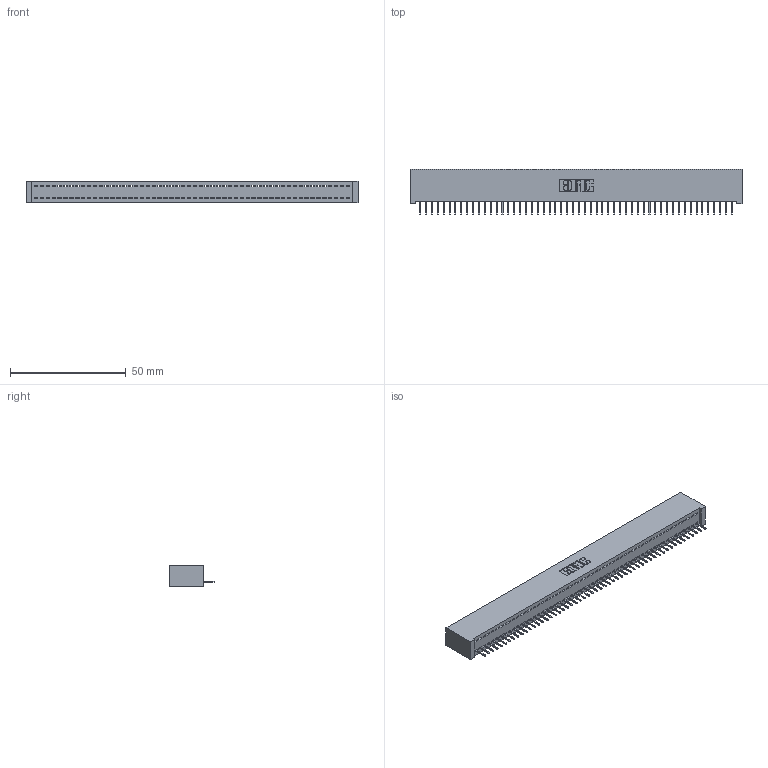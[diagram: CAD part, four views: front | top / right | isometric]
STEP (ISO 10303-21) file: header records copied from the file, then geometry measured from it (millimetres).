
FILE_DESCRIPTION (( 'STEP AP203' ), '1' );
FILE_NAME ('342-054-524-101.STEP', '2019-10-03T02:57:07', ( '' ), ( '' ), 'SwSTEP 2.0', 'SolidWorks 2016', '' );
FILE_SCHEMA (( 'CONFIG_CONTROL_DESIGN' ));
Length unit declared in the file: inch
Products named in the file (3): 342 Part_Lugless; 345-292-001_345-293-124; 342-054-524-101
Assembly tree (55 placements, depth 2):
  342-054-524-101
    342 Part_Lugless
    345-292-001_345-293-124  x54
Bounding box: 143.41 x 19.69 x 9.4 mm (x, y, z)
Volume: 12813.9 mm3; surface area: 18701.4 mm2
Topology: 55 solids, 55 shells, 3450 faces, 9995 edges, 6446 vertices
Faces by surface type: plane 2654, cylinder 796
Entity records: 31125 total; most frequent: CARTESIAN_POINT 5372, ORIENTED_EDGE 5362, DIRECTION 4501, EDGE_CURVE 2681, LINE 2565, VECTOR 2565, VERTEX_POINT 1782, AXIS2_PLACEMENT_3D 968
